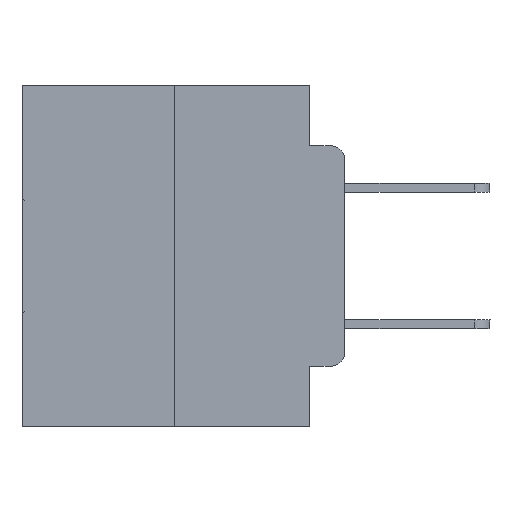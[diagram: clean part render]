
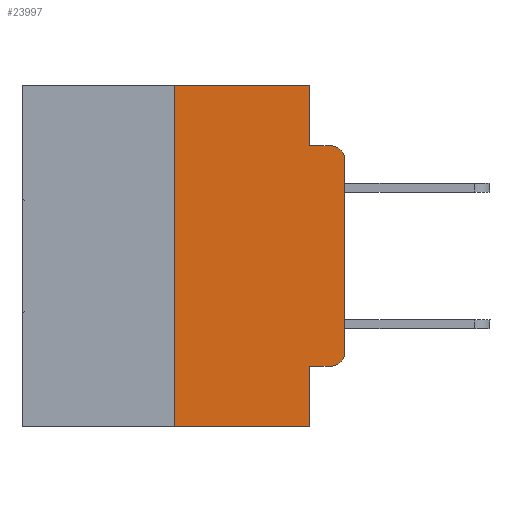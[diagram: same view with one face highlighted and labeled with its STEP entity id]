
A CAD part, left-side view. The second image highlights one B-rep face of the part: STEP entity #23997.
In plain terms, the highlighted planar face has unit normal (-1, 0, 0).
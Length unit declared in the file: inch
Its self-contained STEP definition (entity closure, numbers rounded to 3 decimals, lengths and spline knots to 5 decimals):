
#127 = LINE ( 'NONE', #19449, #7385 ) ;
#320 = DIRECTION ( 'NONE',  ( 0., 0., -1. ) ) ;
#324 = CIRCLE ( 'NONE', #21066, 0.02 ) ;
#1093 = LINE ( 'NONE', #19798, #21211 ) ;
#1203 = AXIS2_PLACEMENT_3D ( 'NONE', #28831, #5730, #320 ) ;
#1227 = LINE ( 'NONE', #29422, #19226 ) ;
#1239 = VERTEX_POINT ( 'NONE', #8988 ) ;
#1347 = LINE ( 'NONE', #8286, #4803 ) ;
#1703 = EDGE_CURVE ( 'NONE', #27574, #20025, #1227, .T. ) ;
#2615 = VERTEX_POINT ( 'NONE', #27120 ) ;
#2633 = DIRECTION ( 'NONE',  ( 0., -1., 0. ) ) ;
#3271 = VECTOR ( 'NONE', #3903, 39.37008 ) ;
#3338 = EDGE_CURVE ( 'NONE', #2615, #22252, #7309, .T. ) ;
#3903 = DIRECTION ( 'NONE',  ( 0., 0., -1. ) ) ;
#4236 = EDGE_CURVE ( 'NONE', #14101, #1239, #324, .T. ) ;
#4314 = EDGE_CURVE ( 'NONE', #21026, #27574, #1347, .T. ) ;
#4402 = CARTESIAN_POINT ( 'NONE',  ( 0., 0.051, 0. ) ) ;
#4803 = VECTOR ( 'NONE', #17730, 39.37008 ) ;
#5310 = ORIENTED_EDGE ( 'NONE', *, *, #19527, .T. ) ;
#5420 = LINE ( 'NONE', #12060, #13466 ) ;
#5574 = CARTESIAN_POINT ( 'NONE',  ( 0., 0., -0.1085 ) ) ;
#5730 = DIRECTION ( 'NONE',  ( 1., 0., 0. ) ) ;
#6878 = EDGE_CURVE ( 'NONE', #1239, #21850, #1093, .T. ) ;
#7309 = LINE ( 'NONE', #14921, #9641 ) ;
#7385 = VECTOR ( 'NONE', #11731, 39.37008 ) ;
#8036 = FACE_OUTER_BOUND ( 'NONE', #30313, .T. ) ;
#8286 = CARTESIAN_POINT ( 'NONE',  ( 0., 0.25, 0. ) ) ;
#8289 = ORIENTED_EDGE ( 'NONE', *, *, #21899, .T. ) ;
#8429 = AXIS2_PLACEMENT_3D ( 'NONE', #23111, #16635, #11689 ) ;
#8988 = CARTESIAN_POINT ( 'NONE',  ( 0., 0., -0.3915 ) ) ;
#9641 = VECTOR ( 'NONE', #24270, 39.37008 ) ;
#9994 = CARTESIAN_POINT ( 'NONE',  ( 0., 0.02, -0.3915 ) ) ;
#10254 = ORIENTED_EDGE ( 'NONE', *, *, #25565, .F. ) ;
#11079 = CARTESIAN_POINT ( 'NONE',  ( 0., 0.25, 0. ) ) ;
#11122 = DIRECTION ( 'NONE',  ( 0., -1., 0. ) ) ;
#11392 = CIRCLE ( 'NONE', #8429, 0.02 ) ;
#11689 = DIRECTION ( 'NONE',  ( 0., 0., -1. ) ) ;
#11731 = DIRECTION ( 'NONE',  ( 0., 0., -1. ) ) ;
#12060 = CARTESIAN_POINT ( 'NONE',  ( 0., 0.473, -0.5 ) ) ;
#13466 = VECTOR ( 'NONE', #14718, 39.37008 ) ;
#14101 = VERTEX_POINT ( 'NONE', #23427 ) ;
#14579 = VERTEX_POINT ( 'NONE', #19072 ) ;
#14718 = DIRECTION ( 'NONE',  ( 0., -1., 0. ) ) ;
#14921 = CARTESIAN_POINT ( 'NONE',  ( 0., 0.051, -0.0885 ) ) ;
#16635 = DIRECTION ( 'NONE',  ( -1., 0., 0. ) ) ;
#16963 = DIRECTION ( 'NONE',  ( 0., 0., -1. ) ) ;
#17017 = DIRECTION ( 'NONE',  ( 0., 0., 1. ) ) ;
#17730 = DIRECTION ( 'NONE',  ( 0., 0., 1. ) ) ;
#17963 = CARTESIAN_POINT ( 'NONE',  ( 0., 0.051, 0. ) ) ;
#18974 = ORIENTED_EDGE ( 'NONE', *, *, #3338, .F. ) ;
#19072 = CARTESIAN_POINT ( 'NONE',  ( 0., 0.051, -0.5 ) ) ;
#19083 = EDGE_CURVE ( 'NONE', #20025, #2615, #127, .T. ) ;
#19226 = VECTOR ( 'NONE', #11122, 39.37008 ) ;
#19261 = CARTESIAN_POINT ( 'NONE',  ( 0., 0.25, -0.5 ) ) ;
#19449 = CARTESIAN_POINT ( 'NONE',  ( 0., 0.051, 0. ) ) ;
#19467 = VERTEX_POINT ( 'NONE', #29387 ) ;
#19527 = EDGE_CURVE ( 'NONE', #21850, #22252, #11392, .T. ) ;
#19633 = VECTOR ( 'NONE', #2633, 39.37008 ) ;
#19798 = CARTESIAN_POINT ( 'NONE',  ( 0., 0., 0. ) ) ;
#20025 = VERTEX_POINT ( 'NONE', #4402 ) ;
#20419 = LINE ( 'NONE', #17963, #3271 ) ;
#20526 = ORIENTED_EDGE ( 'NONE', *, *, #4236, .T. ) ;
#20670 = ORIENTED_EDGE ( 'NONE', *, *, #6878, .T. ) ;
#21026 = VERTEX_POINT ( 'NONE', #19261 ) ;
#21066 = AXIS2_PLACEMENT_3D ( 'NONE', #9994, #24155, #16963 ) ;
#21211 = VECTOR ( 'NONE', #17017, 39.37008 ) ;
#21394 = ORIENTED_EDGE ( 'NONE', *, *, #4314, .F. ) ;
#21850 = VERTEX_POINT ( 'NONE', #5574 ) ;
#21899 = EDGE_CURVE ( 'NONE', #21026, #14579, #5420, .T. ) ;
#22252 = VERTEX_POINT ( 'NONE', #28198 ) ;
#23111 = CARTESIAN_POINT ( 'NONE',  ( 0., 0.02, -0.1085 ) ) ;
#23329 = ORIENTED_EDGE ( 'NONE', *, *, #1703, .F. ) ;
#23427 = CARTESIAN_POINT ( 'NONE',  ( 0., 0.02, -0.4115 ) ) ;
#23740 = LINE ( 'NONE', #24188, #19633 ) ;
#23997 = ADVANCED_FACE ( 'NONE', ( #8036 ), #26833, .F. ) ;
#24155 = DIRECTION ( 'NONE',  ( -1., 0., 0. ) ) ;
#24188 = CARTESIAN_POINT ( 'NONE',  ( 0., 0.051, -0.4115 ) ) ;
#24270 = DIRECTION ( 'NONE',  ( 0., -1., 0. ) ) ;
#25565 = EDGE_CURVE ( 'NONE', #19467, #14579, #20419, .T. ) ;
#26833 = PLANE ( 'NONE',  #1203 ) ;
#27120 = CARTESIAN_POINT ( 'NONE',  ( 0., 0.051, -0.0885 ) ) ;
#27372 = ORIENTED_EDGE ( 'NONE', *, *, #28316, .T. ) ;
#27574 = VERTEX_POINT ( 'NONE', #11079 ) ;
#28198 = CARTESIAN_POINT ( 'NONE',  ( 0., 0.02, -0.0885 ) ) ;
#28316 = EDGE_CURVE ( 'NONE', #19467, #14101, #23740, .T. ) ;
#28831 = CARTESIAN_POINT ( 'NONE',  ( 0., 0.473, 0. ) ) ;
#29387 = CARTESIAN_POINT ( 'NONE',  ( 0., 0.051, -0.4115 ) ) ;
#29422 = CARTESIAN_POINT ( 'NONE',  ( 0., 0.473, 0. ) ) ;
#29643 = ORIENTED_EDGE ( 'NONE', *, *, #19083, .F. ) ;
#30313 = EDGE_LOOP ( 'NONE', ( #20670, #5310, #18974, #29643, #23329, #21394, #8289, #10254, #27372, #20526 ) ) ;
